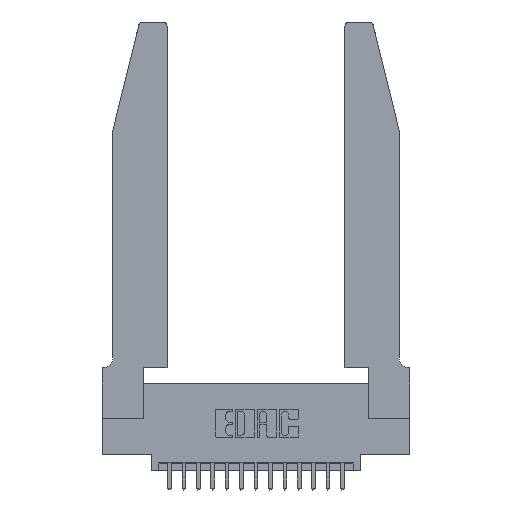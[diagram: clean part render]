
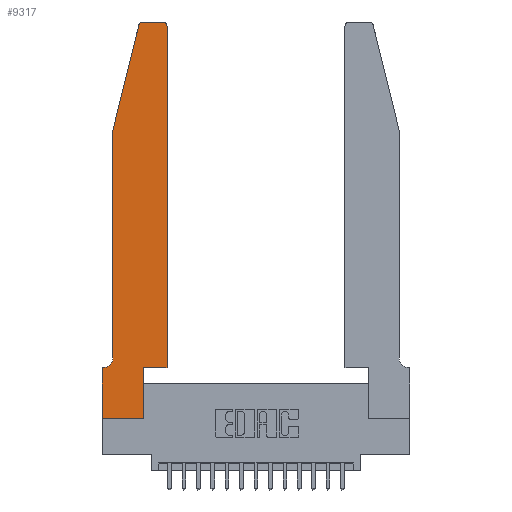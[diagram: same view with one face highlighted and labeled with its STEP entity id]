
A CAD part, top view. The second image highlights one B-rep face of the part: STEP entity #9317.
In plain terms, the highlighted planar face has unit normal (0, 0, 1).
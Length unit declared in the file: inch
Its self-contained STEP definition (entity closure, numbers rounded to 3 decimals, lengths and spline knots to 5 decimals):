
#78 = VERTEX_POINT ( 'NONE', #17482 ) ;
#219 = LINE ( 'NONE', #918, #2816 ) ;
#465 = EDGE_LOOP ( 'NONE', ( #1481, #1030, #5610, #10082, #3197, #14620, #17812, #9024, #2933, #6932, #3913, #9472 ) ) ;
#622 = LINE ( 'NONE', #16344, #11964 ) ;
#918 = CARTESIAN_POINT ( 'NONE',  ( 0.2865, 0.35, 0.37 ) ) ;
#1030 = ORIENTED_EDGE ( 'NONE', *, *, #19022, .T. ) ;
#1410 = VECTOR ( 'NONE', #11585, 39.37008 ) ;
#1481 = ORIENTED_EDGE ( 'NONE', *, *, #14034, .T. ) ;
#1881 = EDGE_CURVE ( 'NONE', #16426, #6999, #4305, .T. ) ;
#1888 = CARTESIAN_POINT ( 'NONE',  ( 0., 0.35, 0.37 ) ) ;
#1967 = VECTOR ( 'NONE', #18354, 39.37008 ) ;
#2147 = AXIS2_PLACEMENT_3D ( 'NONE', #13567, #4748, #15004 ) ;
#2159 = CARTESIAN_POINT ( 'NONE',  ( 0.0755, 2., 0.37 ) ) ;
#2286 = DIRECTION ( 'NONE',  ( 0., 0., 1. ) ) ;
#2504 = EDGE_CURVE ( 'NONE', #7064, #15313, #17984, .T. ) ;
#2816 = VECTOR ( 'NONE', #14127, 39.37008 ) ;
#2921 = VERTEX_POINT ( 'NONE', #8807 ) ;
#2933 = ORIENTED_EDGE ( 'NONE', *, *, #5597, .T. ) ;
#3070 = EDGE_CURVE ( 'NONE', #2921, #9863, #9353, .T. ) ;
#3104 = CARTESIAN_POINT ( 'NONE',  ( 0.4505, 0.35, 0.37 ) ) ;
#3143 = DIRECTION ( 'NONE',  ( -1., 0., 0. ) ) ;
#3197 = ORIENTED_EDGE ( 'NONE', *, *, #8827, .T. ) ;
#3913 = ORIENTED_EDGE ( 'NONE', *, *, #2504, .T. ) ;
#4242 = DIRECTION ( 'NONE',  ( -0.239, -0.971, 0. ) ) ;
#4305 = LINE ( 'NONE', #2159, #7765 ) ;
#4353 = LINE ( 'NONE', #10134, #18529 ) ;
#4651 = CARTESIAN_POINT ( 'NONE',  ( 0., 0., 0.37 ) ) ;
#4748 = DIRECTION ( 'NONE',  ( 0., 0., 1. ) ) ;
#5184 = CARTESIAN_POINT ( 'NONE',  ( 0., 0., 0.37 ) ) ;
#5597 = EDGE_CURVE ( 'NONE', #9866, #16377, #219, .T. ) ;
#5610 = ORIENTED_EDGE ( 'NONE', *, *, #10177, .T. ) ;
#5778 = CIRCLE ( 'NONE', #2147, 0.03 ) ;
#6047 = AXIS2_PLACEMENT_3D ( 'NONE', #8460, #18629, #9961 ) ;
#6623 = CARTESIAN_POINT ( 'NONE',  ( 0.4505, 0.35, 0.37 ) ) ;
#6789 = DIRECTION ( 'NONE',  ( 0., -1., 0. ) ) ;
#6932 = ORIENTED_EDGE ( 'NONE', *, *, #14642, .T. ) ;
#6999 = VERTEX_POINT ( 'NONE', #13850 ) ;
#7064 = VERTEX_POINT ( 'NONE', #6623 ) ;
#7550 = DIRECTION ( 'NONE',  ( 0., -1., 0. ) ) ;
#7681 = CARTESIAN_POINT ( 'NONE',  ( 0., 0., 0.37 ) ) ;
#7765 = VECTOR ( 'NONE', #6789, 39.37008 ) ;
#7828 = DIRECTION ( 'NONE',  ( 0., 0., 1. ) ) ;
#8132 = DIRECTION ( 'NONE',  ( 1., 0., 0. ) ) ;
#8460 = CARTESIAN_POINT ( 'NONE',  ( 0.0055, 0.42, 0.37 ) ) ;
#8585 = DIRECTION ( 'NONE',  ( -1., 0., 0. ) ) ;
#8786 = CARTESIAN_POINT ( 'NONE',  ( 0.4205, 2.75, 0.37 ) ) ;
#8807 = CARTESIAN_POINT ( 'NONE',  ( 0., 0.35, 0.37 ) ) ;
#8827 = EDGE_CURVE ( 'NONE', #6999, #17550, #12680, .T. ) ;
#9024 = ORIENTED_EDGE ( 'NONE', *, *, #15665, .T. ) ;
#9317 = ADVANCED_FACE ( 'NONE', ( #15598 ), #13675, .T. ) ;
#9353 = LINE ( 'NONE', #7681, #16183 ) ;
#9472 = ORIENTED_EDGE ( 'NONE', *, *, #16818, .T. ) ;
#9863 = VERTEX_POINT ( 'NONE', #4651 ) ;
#9866 = VERTEX_POINT ( 'NONE', #14916 ) ;
#9926 = CARTESIAN_POINT ( 'NONE',  ( 0.0055, 0.35, 0.37 ) ) ;
#9961 = DIRECTION ( 'NONE',  ( -1., 0., 0. ) ) ;
#10082 = ORIENTED_EDGE ( 'NONE', *, *, #1881, .T. ) ;
#10134 = CARTESIAN_POINT ( 'NONE',  ( 0.0755, 2., 0.37 ) ) ;
#10177 = EDGE_CURVE ( 'NONE', #78, #16426, #4353, .T. ) ;
#10336 = EDGE_CURVE ( 'NONE', #17550, #2921, #622, .T. ) ;
#11131 = CARTESIAN_POINT ( 'NONE',  ( 0.4205, 2.72, 0.37 ) ) ;
#11394 = AXIS2_PLACEMENT_3D ( 'NONE', #11131, #2286, #12604 ) ;
#11585 = DIRECTION ( 'NONE',  ( 1., 0., 0. ) ) ;
#11872 = VECTOR ( 'NONE', #8132, 39.37008 ) ;
#11964 = VECTOR ( 'NONE', #3143, 39.37008 ) ;
#12242 = AXIS2_PLACEMENT_3D ( 'NONE', #1888, #7828, #17995 ) ;
#12315 = LINE ( 'NONE', #5184, #11872 ) ;
#12604 = DIRECTION ( 'NONE',  ( 1., 0., 0. ) ) ;
#12680 = CIRCLE ( 'NONE', #6047, 0.07 ) ;
#13039 = VERTEX_POINT ( 'NONE', #14754 ) ;
#13216 = CARTESIAN_POINT ( 'NONE',  ( 0.4505, 2.72, 0.37 ) ) ;
#13567 = CARTESIAN_POINT ( 'NONE',  ( 0.284, 2.72, 0.37 ) ) ;
#13675 = PLANE ( 'NONE',  #12242 ) ;
#13850 = CARTESIAN_POINT ( 'NONE',  ( 0.0755, 0.42, 0.37 ) ) ;
#14034 = EDGE_CURVE ( 'NONE', #14138, #13039, #15906, .T. ) ;
#14127 = DIRECTION ( 'NONE',  ( 0., 1., 0. ) ) ;
#14138 = VERTEX_POINT ( 'NONE', #8786 ) ;
#14377 = CARTESIAN_POINT ( 'NONE',  ( 0.0755, 2., 0.37 ) ) ;
#14620 = ORIENTED_EDGE ( 'NONE', *, *, #10336, .T. ) ;
#14642 = EDGE_CURVE ( 'NONE', #16377, #7064, #17013, .T. ) ;
#14754 = CARTESIAN_POINT ( 'NONE',  ( 0.284, 2.75, 0.37 ) ) ;
#14916 = CARTESIAN_POINT ( 'NONE',  ( 0.2865, 0., 0.37 ) ) ;
#15004 = DIRECTION ( 'NONE',  ( 1., 0., 0. ) ) ;
#15313 = VERTEX_POINT ( 'NONE', #13216 ) ;
#15453 = VECTOR ( 'NONE', #8585, 39.37008 ) ;
#15598 = FACE_OUTER_BOUND ( 'NONE', #465, .T. ) ;
#15665 = EDGE_CURVE ( 'NONE', #9863, #9866, #12315, .T. ) ;
#15858 = CARTESIAN_POINT ( 'NONE',  ( 0.2605, 2.75, 0.37 ) ) ;
#15906 = LINE ( 'NONE', #15858, #15453 ) ;
#16183 = VECTOR ( 'NONE', #7550, 39.37008 ) ;
#16344 = CARTESIAN_POINT ( 'NONE',  ( 0.0755, 0.35, 0.37 ) ) ;
#16349 = CIRCLE ( 'NONE', #11394, 0.03 ) ;
#16377 = VERTEX_POINT ( 'NONE', #17466 ) ;
#16426 = VERTEX_POINT ( 'NONE', #14377 ) ;
#16818 = EDGE_CURVE ( 'NONE', #15313, #14138, #16349, .T. ) ;
#17013 = LINE ( 'NONE', #18801, #1410 ) ;
#17466 = CARTESIAN_POINT ( 'NONE',  ( 0.2865, 0.35, 0.37 ) ) ;
#17482 = CARTESIAN_POINT ( 'NONE',  ( 0.25487, 2.72718, 0.37 ) ) ;
#17550 = VERTEX_POINT ( 'NONE', #9926 ) ;
#17812 = ORIENTED_EDGE ( 'NONE', *, *, #3070, .T. ) ;
#17984 = LINE ( 'NONE', #3104, #1967 ) ;
#17995 = DIRECTION ( 'NONE',  ( 1., 0., 0. ) ) ;
#18354 = DIRECTION ( 'NONE',  ( 0., 1., 0. ) ) ;
#18529 = VECTOR ( 'NONE', #4242, 39.37008 ) ;
#18629 = DIRECTION ( 'NONE',  ( 0., 0., -1. ) ) ;
#18801 = CARTESIAN_POINT ( 'NONE',  ( 0.4505, 0.35, 0.37 ) ) ;
#19022 = EDGE_CURVE ( 'NONE', #13039, #78, #5778, .T. ) ;
